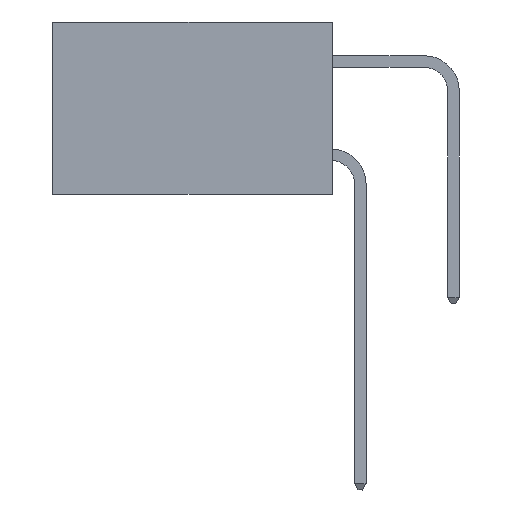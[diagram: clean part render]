
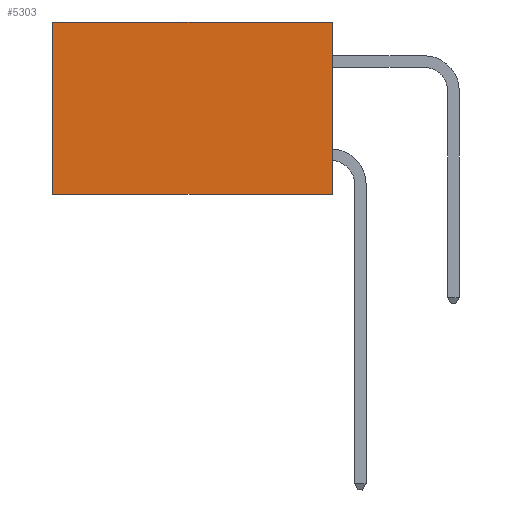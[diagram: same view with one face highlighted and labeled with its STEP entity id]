
A CAD part, left-side view. The second image highlights one B-rep face of the part: STEP entity #5303.
In plain terms, the highlighted planar face has unit normal (-1, 0, 0).
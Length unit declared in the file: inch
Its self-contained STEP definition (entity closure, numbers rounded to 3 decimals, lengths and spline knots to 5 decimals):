
#623 = ORIENTED_EDGE ( 'NONE', *, *, #20385, .T. ) ;
#890 = CARTESIAN_POINT ( 'NONE',  ( 0.2615, 0., -0.37 ) ) ;
#1561 = LINE ( 'NONE', #22364, #9518 ) ;
#2691 = ORIENTED_EDGE ( 'NONE', *, *, #25118, .F. ) ;
#3551 = DIRECTION ( 'NONE',  ( 0., 0., -1. ) ) ;
#5303 = ADVANCED_FACE ( 'NONE', ( #23062 ), #14440, .F. ) ;
#6252 = CARTESIAN_POINT ( 'NONE',  ( 0.2615, 0., -0.37 ) ) ;
#6511 = EDGE_CURVE ( 'NONE', #9498, #25114, #18284, .T. ) ;
#7396 = CARTESIAN_POINT ( 'NONE',  ( 0.2615, 0.6, -0.37 ) ) ;
#7780 = LINE ( 'NONE', #26338, #20746 ) ;
#8799 = EDGE_LOOP ( 'NONE', ( #18434, #22334, #2691, #623 ) ) ;
#9498 = VERTEX_POINT ( 'NONE', #16178 ) ;
#9518 = VECTOR ( 'NONE', #11562, 39.37008 ) ;
#10831 = AXIS2_PLACEMENT_3D ( 'NONE', #6252, #12658, #16743 ) ;
#11537 = CARTESIAN_POINT ( 'NONE',  ( 0.2615, 0., 0. ) ) ;
#11562 = DIRECTION ( 'NONE',  ( 0., 1., 0. ) ) ;
#11638 = VECTOR ( 'NONE', #17944, 39.37008 ) ;
#12053 = CARTESIAN_POINT ( 'NONE',  ( 0.2615, 0., 0. ) ) ;
#12658 = DIRECTION ( 'NONE',  ( 1., 0., 0. ) ) ;
#14382 = VECTOR ( 'NONE', #3551, 39.37008 ) ;
#14440 = PLANE ( 'NONE',  #10831 ) ;
#16078 = DIRECTION ( 'NONE',  ( 0., 0., -1. ) ) ;
#16178 = CARTESIAN_POINT ( 'NONE',  ( 0.2615, 0.6, 0. ) ) ;
#16743 = DIRECTION ( 'NONE',  ( 0., 0., -1. ) ) ;
#17944 = DIRECTION ( 'NONE',  ( 0., 1., 0. ) ) ;
#18284 = LINE ( 'NONE', #26497, #14382 ) ;
#18434 = ORIENTED_EDGE ( 'NONE', *, *, #6511, .T. ) ;
#20385 = EDGE_CURVE ( 'NONE', #21340, #9498, #22465, .T. ) ;
#20746 = VECTOR ( 'NONE', #16078, 39.37008 ) ;
#20897 = EDGE_CURVE ( 'NONE', #26412, #25114, #1561, .T. ) ;
#21340 = VERTEX_POINT ( 'NONE', #12053 ) ;
#22334 = ORIENTED_EDGE ( 'NONE', *, *, #20897, .F. ) ;
#22364 = CARTESIAN_POINT ( 'NONE',  ( 0.2615, 0., -0.37 ) ) ;
#22465 = LINE ( 'NONE', #11537, #11638 ) ;
#23062 = FACE_OUTER_BOUND ( 'NONE', #8799, .T. ) ;
#25114 = VERTEX_POINT ( 'NONE', #7396 ) ;
#25118 = EDGE_CURVE ( 'NONE', #21340, #26412, #7780, .T. ) ;
#26338 = CARTESIAN_POINT ( 'NONE',  ( 0.2615, 0., -0.37 ) ) ;
#26412 = VERTEX_POINT ( 'NONE', #890 ) ;
#26497 = CARTESIAN_POINT ( 'NONE',  ( 0.2615, 0.6, -0.37 ) ) ;
